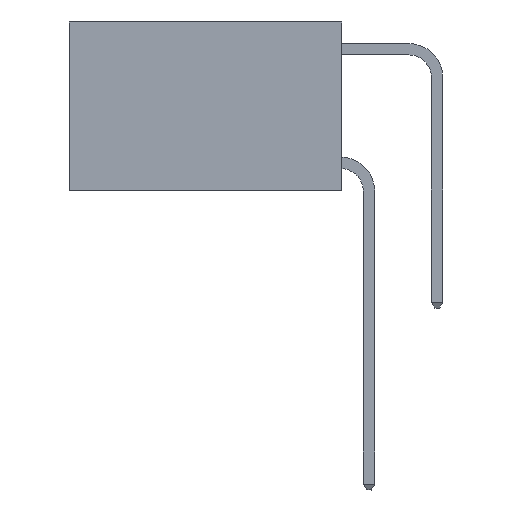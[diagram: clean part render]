
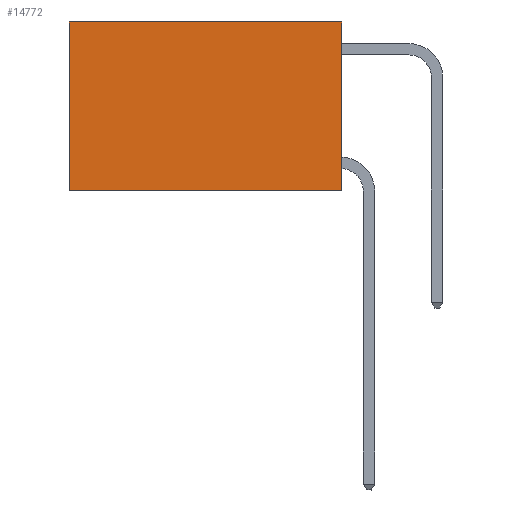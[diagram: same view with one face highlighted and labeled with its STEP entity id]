
A CAD part, left-side view. The second image highlights one B-rep face of the part: STEP entity #14772.
In plain terms, the highlighted planar face has unit normal (-1, 0, 0).
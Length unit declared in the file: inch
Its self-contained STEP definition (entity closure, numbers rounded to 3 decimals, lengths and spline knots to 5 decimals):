
#518 = DIRECTION ( 'NONE',  ( 0., 0., -1. ) ) ;
#853 = VECTOR ( 'NONE', #6355, 39.37008 ) ;
#1520 = VERTEX_POINT ( 'NONE', #11808 ) ;
#1632 = VERTEX_POINT ( 'NONE', #10867 ) ;
#2066 = ORIENTED_EDGE ( 'NONE', *, *, #7354, .F. ) ;
#2135 = EDGE_CURVE ( 'NONE', #6893, #12676, #3472, .T. ) ;
#2506 = LINE ( 'NONE', #3760, #9272 ) ;
#3472 = LINE ( 'NONE', #6377, #853 ) ;
#3760 = CARTESIAN_POINT ( 'NONE',  ( 0.2625, 0., 0. ) ) ;
#3807 = LINE ( 'NONE', #5738, #14367 ) ;
#3971 = EDGE_CURVE ( 'NONE', #1520, #12676, #3807, .T. ) ;
#5605 = ORIENTED_EDGE ( 'NONE', *, *, #2135, .F. ) ;
#5738 = CARTESIAN_POINT ( 'NONE',  ( 0.2625, 0.6, 0. ) ) ;
#6049 = EDGE_LOOP ( 'NONE', ( #8337, #5605, #2066, #13812 ) ) ;
#6355 = DIRECTION ( 'NONE',  ( 0., 1., 0. ) ) ;
#6377 = CARTESIAN_POINT ( 'NONE',  ( 0.2625, 0., -0.37 ) ) ;
#6862 = PLANE ( 'NONE',  #12797 ) ;
#6893 = VERTEX_POINT ( 'NONE', #15462 ) ;
#7354 = EDGE_CURVE ( 'NONE', #1632, #6893, #2506, .T. ) ;
#7490 = CARTESIAN_POINT ( 'NONE',  ( 0.2625, 0., 0. ) ) ;
#8139 = DIRECTION ( 'NONE',  ( 1., 0., 0. ) ) ;
#8337 = ORIENTED_EDGE ( 'NONE', *, *, #3971, .T. ) ;
#9272 = VECTOR ( 'NONE', #13968, 39.37008 ) ;
#9618 = LINE ( 'NONE', #7490, #9997 ) ;
#9997 = VECTOR ( 'NONE', #16424, 39.37008 ) ;
#10867 = CARTESIAN_POINT ( 'NONE',  ( 0.2625, 0., 0. ) ) ;
#11310 = EDGE_CURVE ( 'NONE', #1632, #1520, #9618, .T. ) ;
#11808 = CARTESIAN_POINT ( 'NONE',  ( 0.2625, 0.6, 0. ) ) ;
#12676 = VERTEX_POINT ( 'NONE', #14154 ) ;
#12797 = AXIS2_PLACEMENT_3D ( 'NONE', #15801, #8139, #518 ) ;
#13812 = ORIENTED_EDGE ( 'NONE', *, *, #11310, .T. ) ;
#13968 = DIRECTION ( 'NONE',  ( 0., 0., -1. ) ) ;
#14154 = CARTESIAN_POINT ( 'NONE',  ( 0.2625, 0.6, -0.37 ) ) ;
#14367 = VECTOR ( 'NONE', #14663, 39.37008 ) ;
#14663 = DIRECTION ( 'NONE',  ( 0., 0., -1. ) ) ;
#14715 = FACE_OUTER_BOUND ( 'NONE', #6049, .T. ) ;
#14772 = ADVANCED_FACE ( 'NONE', ( #14715 ), #6862, .F. ) ;
#15462 = CARTESIAN_POINT ( 'NONE',  ( 0.2625, 0., -0.37 ) ) ;
#15801 = CARTESIAN_POINT ( 'NONE',  ( 0.2625, 0., 0. ) ) ;
#16424 = DIRECTION ( 'NONE',  ( 0., 1., 0. ) ) ;
